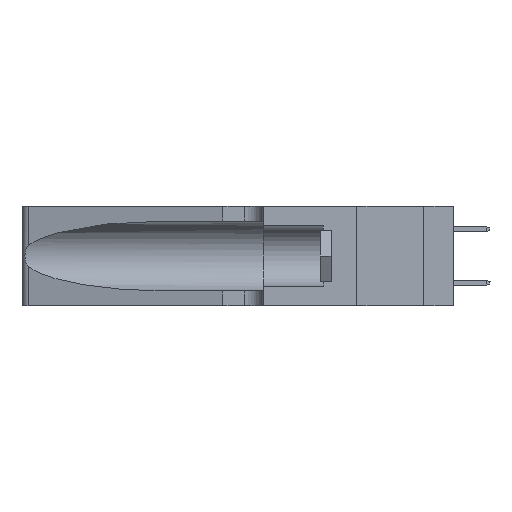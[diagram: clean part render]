
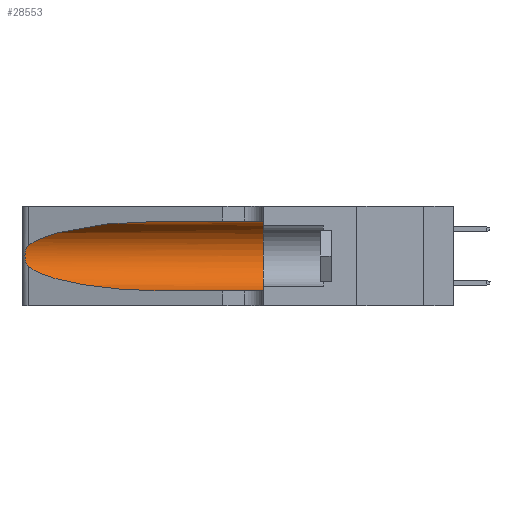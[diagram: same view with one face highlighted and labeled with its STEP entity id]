
A CAD part, left-side view. The second image highlights one B-rep face of the part: STEP entity #28553.
In plain terms, the highlighted cylindrical face has radius 3.308 mm (diameter 6.617 mm), a partial arc.
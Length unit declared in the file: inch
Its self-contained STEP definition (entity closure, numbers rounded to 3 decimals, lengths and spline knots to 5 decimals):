
#382 = CARTESIAN_POINT ( 'NONE',  ( 0.25487, 1.22718, 0.22369 ) ) ;
#1099 = AXIS2_PLACEMENT_3D ( 'NONE', #4331, #17887, #22165 ) ;
#1680 = CIRCLE ( 'NONE', #4483, 0.13025 ) ;
#2066 = CARTESIAN_POINT ( 'NONE',  ( 0.2373, 1.15595, 0.08982 ) ) ;
#2292 = EDGE_CURVE ( 'NONE', #3747, #27760, #1680, .T. ) ;
#3337 = DIRECTION ( 'NONE',  ( 0., -1., 0. ) ) ;
#3419 = CARTESIAN_POINT ( 'NONE',  ( 0.1305, 0.35, 0.05475 ) ) ;
#3644 = EDGE_CURVE ( 'NONE', #24687, #20412, #23736, .T. ) ;
#3747 = VERTEX_POINT ( 'NONE', #20233 ) ;
#3889 = CARTESIAN_POINT ( 'NONE',  ( 0.26075, 1.23896, 0.178 ) ) ;
#3892 = VECTOR ( 'NONE', #3337, 39.37008 ) ;
#4331 = CARTESIAN_POINT ( 'NONE',  ( 0.1305, 1.61858, 0.185 ) ) ;
#4483 = AXIS2_PLACEMENT_3D ( 'NONE', #15961, #20639, #22423 ) ;
#5788 = CARTESIAN_POINT ( 'NONE',  ( 0.26018, 1.23835, 0.19895 ) ) ;
#6213 = VECTOR ( 'NONE', #13041, 39.37008 ) ;
#6945 = CARTESIAN_POINT ( 'NONE',  ( 0.1305, 0.72297, 0.05475 ) ) ;
#7328 = EDGE_CURVE ( 'NONE', #20412, #24859, #10421, .T. ) ;
#7971 = CARTESIAN_POINT ( 'NONE',  ( 0.25639, 1.23184, 0.21858 ) ) ;
#7995 = LINE ( 'NONE', #16893, #3892 ) ;
#8347 = CARTESIAN_POINT ( 'NONE',  ( 0.25487, 1.22718, 0.14631 ) ) ;
#8656 = ORIENTED_EDGE ( 'NONE', *, *, #3644, .T. ) ;
#9556 = CARTESIAN_POINT ( 'NONE',  ( 0.1305, 0.72297, 0.31525 ) ) ;
#9682 = ORIENTED_EDGE ( 'NONE', *, *, #2292, .F. ) ;
#10421 =( BOUNDED_CURVE ( )  B_SPLINE_CURVE ( 3, ( #8347, #2066, #19884, #26480 ),
 .UNSPECIFIED., .F., .T. ) 
 B_SPLINE_CURVE_WITH_KNOTS ( ( 4, 4 ),
 ( 3.44316, 4.71239 ),
 .UNSPECIFIED. ) 
 CURVE ( )  GEOMETRIC_REPRESENTATION_ITEM ( )  RATIONAL_B_SPLINE_CURVE ( ( 1., 0.87, 0.87, 1. ) ) 
 REPRESENTATION_ITEM ( '' )  );
#12155 = EDGE_CURVE ( 'NONE', #24859, #27760, #24417, .T. ) ;
#12330 = EDGE_CURVE ( 'NONE', #27812, #3747, #7995, .T. ) ;
#12355 = CARTESIAN_POINT ( 'NONE',  ( 0.25555, 1.22994, 0.2215 ) ) ;
#12513 = CARTESIAN_POINT ( 'NONE',  ( 0.25639, 1.23186, 0.15144 ) ) ;
#12656 = CARTESIAN_POINT ( 'NONE',  ( 0.25487, 1.22718, 0.22369 ) ) ;
#13041 = DIRECTION ( 'NONE',  ( 0., -1., 0. ) ) ;
#13477 = CARTESIAN_POINT ( 'NONE',  ( 0.1305, 0.72297, 0.31525 ) ) ;
#13844 = EDGE_CURVE ( 'NONE', #27812, #24687, #21650, .T. ) ;
#14887 = CARTESIAN_POINT ( 'NONE',  ( 0.25487, 1.22718, 0.14631 ) ) ;
#15406 = FACE_OUTER_BOUND ( 'NONE', #26168, .T. ) ;
#15961 = CARTESIAN_POINT ( 'NONE',  ( 0.1305, 0.35, 0.185 ) ) ;
#16138 = CARTESIAN_POINT ( 'NONE',  ( 0.2373, 1.15595, 0.28018 ) ) ;
#16893 = CARTESIAN_POINT ( 'NONE',  ( 0.1305, 1.61858, 0.31525 ) ) ;
#17887 = DIRECTION ( 'NONE',  ( 0., -1., 0. ) ) ;
#18395 = ORIENTED_EDGE ( 'NONE', *, *, #13844, .T. ) ;
#19884 = CARTESIAN_POINT ( 'NONE',  ( 0.18966, 0.96281, 0.05475 ) ) ;
#20126 = ORIENTED_EDGE ( 'NONE', *, *, #12330, .F. ) ;
#20233 = CARTESIAN_POINT ( 'NONE',  ( 0.1305, 0.35, 0.31525 ) ) ;
#20412 = VERTEX_POINT ( 'NONE', #14887 ) ;
#20639 = DIRECTION ( 'NONE',  ( 0., 1., 0. ) ) ;
#21417 = CARTESIAN_POINT ( 'NONE',  ( 0.25787, 1.23484, 0.2124 ) ) ;
#21553 = CARTESIAN_POINT ( 'NONE',  ( 0.25555, 1.22993, 0.14849 ) ) ;
#21650 =( BOUNDED_CURVE ( )  B_SPLINE_CURVE ( 3, ( #9556, #24917, #16138, #382 ),
 .UNSPECIFIED., .F., .T. ) 
 B_SPLINE_CURVE_WITH_KNOTS ( ( 4, 4 ),
 ( 1.5708, 2.84003 ),
 .UNSPECIFIED. ) 
 CURVE ( )  GEOMETRIC_REPRESENTATION_ITEM ( )  RATIONAL_B_SPLINE_CURVE ( ( 1., 0.87, 0.87, 1. ) ) 
 REPRESENTATION_ITEM ( '' )  );
#22005 = CYLINDRICAL_SURFACE ( 'NONE', #1099, 0.13025 ) ;
#22165 = DIRECTION ( 'NONE',  ( 0., 0., -1. ) ) ;
#22423 = DIRECTION ( 'NONE',  ( 0., 0., 1. ) ) ;
#23736 = B_SPLINE_CURVE_WITH_KNOTS ( 'NONE', 3,
 ( #12656, #12355, #7971, #21417, #28286, #5788, #23892, #3889, #26251, #25805, #25661, #12513, #21553, #28435 ),
 .UNSPECIFIED., .F., .F.,
 ( 4, 2, 2, 2, 2, 2, 4 ),
 ( 0., 0.00027, 0.00053, 0.00107, 0.0016, 0.00187, 0.00214 ),
 .UNSPECIFIED. ) ;
#23892 = CARTESIAN_POINT ( 'NONE',  ( 0.26075, 1.23896, 0.19203 ) ) ;
#24417 = LINE ( 'NONE', #28514, #6213 ) ;
#24687 = VERTEX_POINT ( 'NONE', #27981 ) ;
#24859 = VERTEX_POINT ( 'NONE', #6945 ) ;
#24917 = CARTESIAN_POINT ( 'NONE',  ( 0.18966, 0.96281, 0.31525 ) ) ;
#25154 = ORIENTED_EDGE ( 'NONE', *, *, #12155, .T. ) ;
#25661 = CARTESIAN_POINT ( 'NONE',  ( 0.25789, 1.23486, 0.15765 ) ) ;
#25805 = CARTESIAN_POINT ( 'NONE',  ( 0.25856, 1.23593, 0.16098 ) ) ;
#26168 = EDGE_LOOP ( 'NONE', ( #18395, #8656, #27293, #25154, #9682, #20126 ) ) ;
#26251 = CARTESIAN_POINT ( 'NONE',  ( 0.26017, 1.23833, 0.17102 ) ) ;
#26480 = CARTESIAN_POINT ( 'NONE',  ( 0.1305, 0.72297, 0.05475 ) ) ;
#27293 = ORIENTED_EDGE ( 'NONE', *, *, #7328, .T. ) ;
#27760 = VERTEX_POINT ( 'NONE', #3419 ) ;
#27812 = VERTEX_POINT ( 'NONE', #13477 ) ;
#27981 = CARTESIAN_POINT ( 'NONE',  ( 0.25487, 1.22718, 0.22369 ) ) ;
#28286 = CARTESIAN_POINT ( 'NONE',  ( 0.25854, 1.2359, 0.20912 ) ) ;
#28435 = CARTESIAN_POINT ( 'NONE',  ( 0.25487, 1.22718, 0.14631 ) ) ;
#28514 = CARTESIAN_POINT ( 'NONE',  ( 0.1305, 1.61858, 0.05475 ) ) ;
#28553 = ADVANCED_FACE ( 'NONE', ( #15406 ), #22005, .F. ) ;
